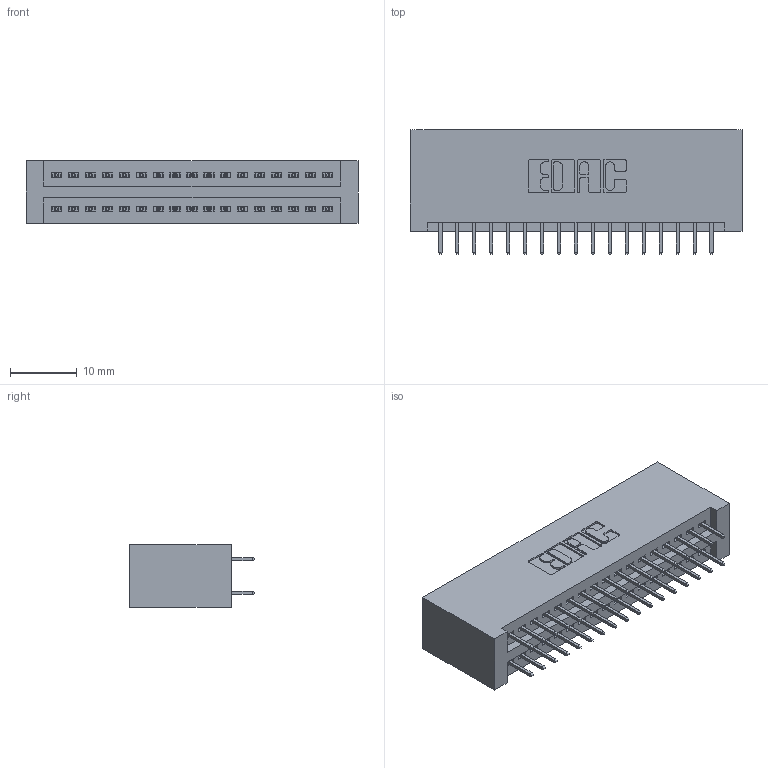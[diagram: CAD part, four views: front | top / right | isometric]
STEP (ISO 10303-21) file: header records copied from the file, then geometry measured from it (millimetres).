
FILE_DESCRIPTION (( 'STEP AP203' ), '1' );
FILE_NAME ('895-034-525-201.STEP', '2020-09-25T21:39:52', ( '' ), ( '' ), 'SwSTEP 2.0', 'SolidWorks 2020', '' );
FILE_SCHEMA (( 'CONFIG_CONTROL_DESIGN' ));
Length unit declared in the file: inch
Products named in the file (3): 845 Part_No Mounting Lugs; 895-034-525-201; 345-292-001_345-293-125
Assembly tree (35 placements, depth 2):
  895-034-525-201
    845 Part_No Mounting Lugs
    345-292-001_345-293-125  x34
Bounding box: 49.78 x 18.72 x 9.4 mm (x, y, z)
Volume: 5164 mm3; surface area: 7283.6 mm2
Topology: 35 solids, 35 shells, 1954 faces, 5519 edges, 3542 vertices
Faces by surface type: plane 1402, cylinder 552
Entity records: 16501 total; most frequent: CARTESIAN_POINT 2788, ORIENTED_EDGE 2722, DIRECTION 2485, EDGE_CURVE 1361, LINE 1173, VECTOR 1173, VERTEX_POINT 902, AXIS2_PLACEMENT_3D 656
